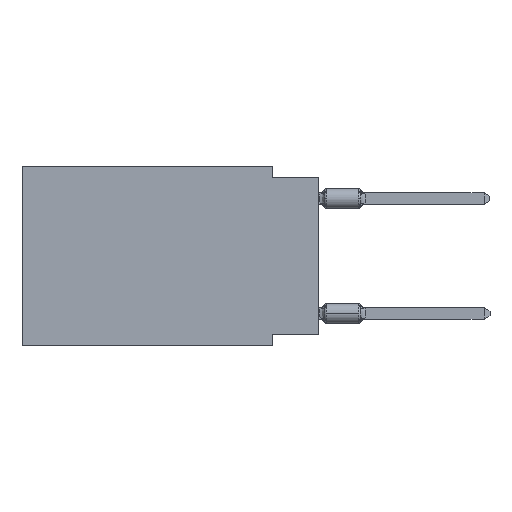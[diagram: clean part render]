
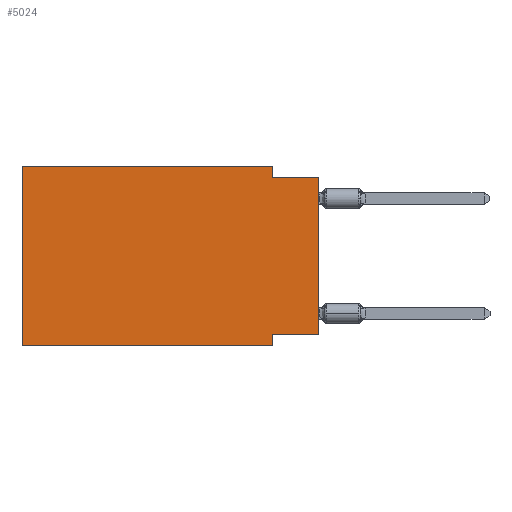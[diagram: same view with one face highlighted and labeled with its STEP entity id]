
A CAD part, left-side view. The second image highlights one B-rep face of the part: STEP entity #5024.
In plain terms, the highlighted planar face has unit normal (-1, 0, 0).
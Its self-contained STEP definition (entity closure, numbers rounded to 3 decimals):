
#33 = CARTESIAN_POINT ( 'NONE',  ( 0., 2.54, -9.271 ) ) ;
#457 = ORIENTED_EDGE ( 'NONE', *, *, #2795, .T. ) ;
#501 = VERTEX_POINT ( 'NONE', #13259 ) ;
#632 = CARTESIAN_POINT ( 'NONE',  ( 0., 0., -0.635 ) ) ;
#673 = CARTESIAN_POINT ( 'NONE',  ( 0., 0., 0. ) ) ;
#713 = DIRECTION ( 'NONE',  ( 0., 1., 0. ) ) ;
#761 = EDGE_CURVE ( 'NONE', #13930, #501, #12939, .T. ) ;
#788 = ORIENTED_EDGE ( 'NONE', *, *, #8667, .F. ) ;
#865 = LINE ( 'NONE', #6525, #5046 ) ;
#870 = ORIENTED_EDGE ( 'NONE', *, *, #12265, .F. ) ;
#930 = DIRECTION ( 'NONE',  ( 0., 0., -1. ) ) ;
#979 = CARTESIAN_POINT ( 'NONE',  ( 0., 16.383, 0. ) ) ;
#1273 = ORIENTED_EDGE ( 'NONE', *, *, #6265, .F. ) ;
#2367 = CARTESIAN_POINT ( 'NONE',  ( 0., 2.54, 0. ) ) ;
#2606 = VERTEX_POINT ( 'NONE', #8159 ) ;
#2659 = LINE ( 'NONE', #632, #12700 ) ;
#2795 = EDGE_CURVE ( 'NONE', #4668, #2606, #2838, .T. ) ;
#2838 = LINE ( 'NONE', #673, #12834 ) ;
#3145 = VECTOR ( 'NONE', #13879, 1000. ) ;
#3615 = VERTEX_POINT ( 'NONE', #33 ) ;
#3953 = PLANE ( 'NONE',  #10061 ) ;
#4131 = LINE ( 'NONE', #10671, #4320 ) ;
#4320 = VECTOR ( 'NONE', #713, 1000. ) ;
#4668 = VERTEX_POINT ( 'NONE', #9005 ) ;
#5024 = ADVANCED_FACE ( 'NONE', ( #9618 ), #3953, .F. ) ;
#5046 = VECTOR ( 'NONE', #930, 1000. ) ;
#5105 = DIRECTION ( 'NONE',  ( 0., 0., 1. ) ) ;
#5360 = DIRECTION ( 'NONE',  ( 0., -1., 0. ) ) ;
#5498 = VERTEX_POINT ( 'NONE', #8059 ) ;
#5745 = EDGE_CURVE ( 'NONE', #10563, #12941, #8405, .T. ) ;
#6063 = DIRECTION ( 'NONE',  ( 0., -1., 0. ) ) ;
#6265 = EDGE_CURVE ( 'NONE', #13930, #10563, #11214, .T. ) ;
#6347 = DIRECTION ( 'NONE',  ( 1., 0., 0. ) ) ;
#6449 = ORIENTED_EDGE ( 'NONE', *, *, #5745, .F. ) ;
#6525 = CARTESIAN_POINT ( 'NONE',  ( 0., 2.54, -9.906 ) ) ;
#6662 = ORIENTED_EDGE ( 'NONE', *, *, #8932, .F. ) ;
#7678 = ORIENTED_EDGE ( 'NONE', *, *, #761, .T. ) ;
#8059 = CARTESIAN_POINT ( 'NONE',  ( 0., 2.54, -0.635 ) ) ;
#8159 = CARTESIAN_POINT ( 'NONE',  ( 0., 0., -0.635 ) ) ;
#8405 = LINE ( 'NONE', #10880, #10068 ) ;
#8667 = EDGE_CURVE ( 'NONE', #3615, #501, #865, .T. ) ;
#8720 = CARTESIAN_POINT ( 'NONE',  ( 0., 16.383, 0. ) ) ;
#8932 = EDGE_CURVE ( 'NONE', #5498, #2606, #2659, .T. ) ;
#9005 = CARTESIAN_POINT ( 'NONE',  ( 0., 0., -9.271 ) ) ;
#9541 = DIRECTION ( 'NONE',  ( 0., 0., -1. ) ) ;
#9618 = FACE_OUTER_BOUND ( 'NONE', #14128, .T. ) ;
#10061 = AXIS2_PLACEMENT_3D ( 'NONE', #13911, #6347, #9541 ) ;
#10068 = VECTOR ( 'NONE', #5360, 1000. ) ;
#10563 = VERTEX_POINT ( 'NONE', #8720 ) ;
#10671 = CARTESIAN_POINT ( 'NONE',  ( 0., 0., -9.271 ) ) ;
#10880 = CARTESIAN_POINT ( 'NONE',  ( 0., 16.383, 0. ) ) ;
#11214 = LINE ( 'NONE', #979, #13799 ) ;
#11232 = EDGE_CURVE ( 'NONE', #12941, #5498, #12267, .T. ) ;
#11405 = ORIENTED_EDGE ( 'NONE', *, *, #11232, .F. ) ;
#12159 = CARTESIAN_POINT ( 'NONE',  ( 0., 16.383, -9.906 ) ) ;
#12191 = VECTOR ( 'NONE', #13275, 1000. ) ;
#12265 = EDGE_CURVE ( 'NONE', #4668, #3615, #4131, .T. ) ;
#12267 = LINE ( 'NONE', #2367, #12191 ) ;
#12700 = VECTOR ( 'NONE', #6063, 1000. ) ;
#12834 = VECTOR ( 'NONE', #5105, 1000. ) ;
#12939 = LINE ( 'NONE', #13075, #3145 ) ;
#12941 = VERTEX_POINT ( 'NONE', #13003 ) ;
#13003 = CARTESIAN_POINT ( 'NONE',  ( 0., 2.54, 0. ) ) ;
#13075 = CARTESIAN_POINT ( 'NONE',  ( 0., 16.383, -9.906 ) ) ;
#13259 = CARTESIAN_POINT ( 'NONE',  ( 0., 2.54, -9.906 ) ) ;
#13263 = DIRECTION ( 'NONE',  ( 0., 0., 1. ) ) ;
#13275 = DIRECTION ( 'NONE',  ( 0., 0., -1. ) ) ;
#13799 = VECTOR ( 'NONE', #13263, 1000. ) ;
#13879 = DIRECTION ( 'NONE',  ( 0., -1., 0. ) ) ;
#13911 = CARTESIAN_POINT ( 'NONE',  ( 0., 16.383, 0. ) ) ;
#13930 = VERTEX_POINT ( 'NONE', #12159 ) ;
#14128 = EDGE_LOOP ( 'NONE', ( #457, #6662, #11405, #6449, #1273, #7678, #788, #870 ) ) ;
